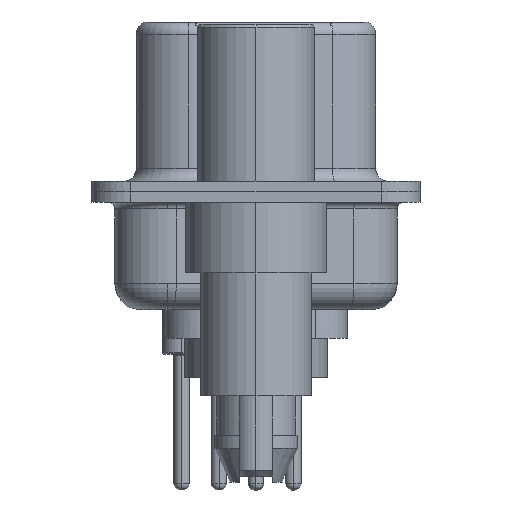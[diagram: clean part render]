
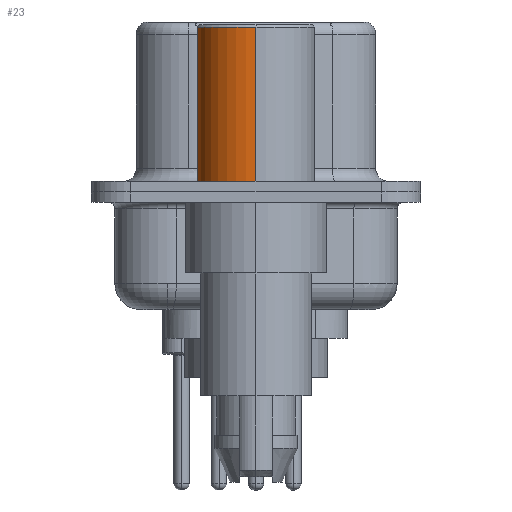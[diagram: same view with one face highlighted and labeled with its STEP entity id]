
A CAD part, left-side view. The second image highlights one B-rep face of the part: STEP entity #23.
In plain terms, the highlighted cylindrical face has radius 2.25 mm (diameter 4.5 mm), a partial arc.
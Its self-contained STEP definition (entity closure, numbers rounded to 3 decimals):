
#23 = ADVANCED_FACE ( 'NONE', ( #11687 ), #15829, .T. ) ;
#536 = AXIS2_PLACEMENT_3D ( 'NONE', #1002, #15054, #3034 ) ;
#1002 = CARTESIAN_POINT ( 'NONE',  ( 0., 0., 0.4 ) ) ;
#1841 = VECTOR ( 'NONE', #14070, 1000. ) ;
#2821 = ORIENTED_EDGE ( 'NONE', *, *, #15577, .F. ) ;
#3034 = DIRECTION ( 'NONE',  ( 1., 0., 0. ) ) ;
#6510 = CIRCLE ( 'NONE', #13667, 2.25 ) ;
#6823 = DIRECTION ( 'NONE',  ( 0., 0., 1. ) ) ;
#6915 = CARTESIAN_POINT ( 'NONE',  ( 0., 0., 0.581 ) ) ;
#7104 = LINE ( 'NONE', #9976, #1841 ) ;
#7425 = ORIENTED_EDGE ( 'NONE', *, *, #19192, .F. ) ;
#8572 = CARTESIAN_POINT ( 'NONE',  ( 0., 0., 6.3 ) ) ;
#9976 = CARTESIAN_POINT ( 'NONE',  ( 2.25, 0., 0.581 ) ) ;
#10063 = CARTESIAN_POINT ( 'NONE',  ( -2.25, 0., 0.581 ) ) ;
#10065 = CARTESIAN_POINT ( 'NONE',  ( 2.25, 0., 6.3 ) ) ;
#10582 = DIRECTION ( 'NONE',  ( 1., 0., 0. ) ) ;
#11066 = ORIENTED_EDGE ( 'NONE', *, *, #21031, .T. ) ;
#11687 = FACE_OUTER_BOUND ( 'NONE', #20637, .T. ) ;
#12322 = EDGE_CURVE ( 'NONE', #16086, #17998, #22543, .T. ) ;
#12403 = VECTOR ( 'NONE', #14609, 1000. ) ;
#13044 = LINE ( 'NONE', #10063, #12403 ) ;
#13070 = CARTESIAN_POINT ( 'NONE',  ( -2.25, 0., 6.3 ) ) ;
#13495 = CARTESIAN_POINT ( 'NONE',  ( 2.25, 0., 0.4 ) ) ;
#13667 = AXIS2_PLACEMENT_3D ( 'NONE', #8572, #22816, #10582 ) ;
#14070 = DIRECTION ( 'NONE',  ( 0., 0., 1. ) ) ;
#14609 = DIRECTION ( 'NONE',  ( 0., 0., 1. ) ) ;
#15054 = DIRECTION ( 'NONE',  ( 0., 0., 1. ) ) ;
#15577 = EDGE_CURVE ( 'NONE', #16086, #17501, #7104, .T. ) ;
#15628 = DIRECTION ( 'NONE',  ( 1., 0., 0. ) ) ;
#15829 = CYLINDRICAL_SURFACE ( 'NONE', #19171, 2.25 ) ;
#15934 = VERTEX_POINT ( 'NONE', #13070 ) ;
#16086 = VERTEX_POINT ( 'NONE', #13495 ) ;
#17501 = VERTEX_POINT ( 'NONE', #10065 ) ;
#17998 = VERTEX_POINT ( 'NONE', #18531 ) ;
#18531 = CARTESIAN_POINT ( 'NONE',  ( -2.25, 0., 0.4 ) ) ;
#19171 = AXIS2_PLACEMENT_3D ( 'NONE', #6915, #6823, #15628 ) ;
#19192 = EDGE_CURVE ( 'NONE', #17501, #15934, #6510, .T. ) ;
#20637 = EDGE_LOOP ( 'NONE', ( #24694, #11066, #7425, #2821 ) ) ;
#21031 = EDGE_CURVE ( 'NONE', #17998, #15934, #13044, .T. ) ;
#22543 = CIRCLE ( 'NONE', #536, 2.25 ) ;
#22816 = DIRECTION ( 'NONE',  ( 0., 0., 1. ) ) ;
#24694 = ORIENTED_EDGE ( 'NONE', *, *, #12322, .T. ) ;
